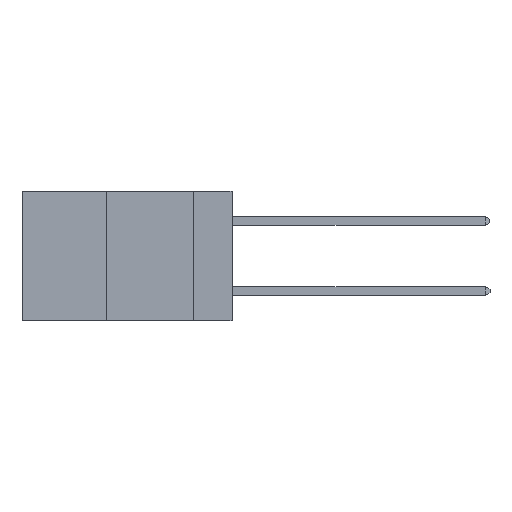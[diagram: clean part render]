
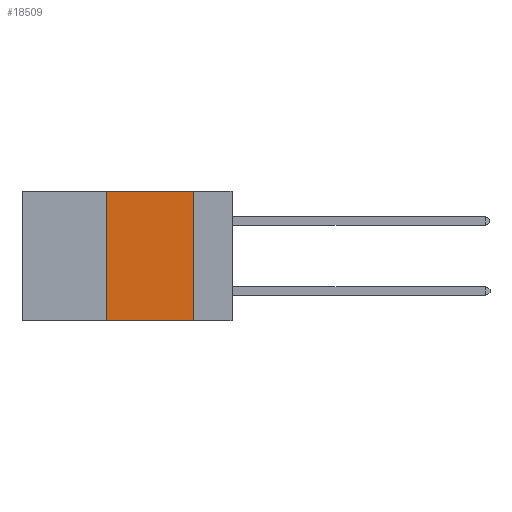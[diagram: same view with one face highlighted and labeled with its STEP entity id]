
A CAD part, left-side view. The second image highlights one B-rep face of the part: STEP entity #18509.
In plain terms, the highlighted planar face has unit normal (-1, 0, 0).
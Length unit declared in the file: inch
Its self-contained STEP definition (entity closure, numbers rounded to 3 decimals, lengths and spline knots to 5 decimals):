
#1529 = EDGE_CURVE ( 'NONE', #11602, #1606, #22416, .T. ) ;
#1606 = VERTEX_POINT ( 'NONE', #14369 ) ;
#1639 = CARTESIAN_POINT ( 'NONE',  ( 0., 0.6, 0. ) ) ;
#1999 = AXIS2_PLACEMENT_3D ( 'NONE', #11808, #15456, #9695 ) ;
#2536 = DIRECTION ( 'NONE',  ( 0., -1., 0. ) ) ;
#2548 = VECTOR ( 'NONE', #16688, 39.37008 ) ;
#2677 = VECTOR ( 'NONE', #16872, 39.37008 ) ;
#2742 = LINE ( 'NONE', #14700, #20110 ) ;
#3551 = ORIENTED_EDGE ( 'NONE', *, *, #13297, .F. ) ;
#3715 = ORIENTED_EDGE ( 'NONE', *, *, #1529, .F. ) ;
#4458 = PLANE ( 'NONE',  #1999 ) ;
#5146 = ORIENTED_EDGE ( 'NONE', *, *, #6043, .T. ) ;
#5927 = CARTESIAN_POINT ( 'NONE',  ( 0., 0.11, 0. ) ) ;
#6043 = EDGE_CURVE ( 'NONE', #11602, #15658, #2742, .T. ) ;
#7690 = VECTOR ( 'NONE', #11779, 39.37008 ) ;
#7703 = FACE_OUTER_BOUND ( 'NONE', #8476, .T. ) ;
#8131 = EDGE_CURVE ( 'NONE', #14094, #15658, #10756, .T. ) ;
#8476 = EDGE_LOOP ( 'NONE', ( #10136, #3551, #3715, #5146 ) ) ;
#9695 = DIRECTION ( 'NONE',  ( 0., 0., -1. ) ) ;
#10136 = ORIENTED_EDGE ( 'NONE', *, *, #8131, .F. ) ;
#10756 = LINE ( 'NONE', #5927, #2677 ) ;
#11602 = VERTEX_POINT ( 'NONE', #12564 ) ;
#11779 = DIRECTION ( 'NONE',  ( 0., 0., 1. ) ) ;
#11801 = LINE ( 'NONE', #1639, #2548 ) ;
#11808 = CARTESIAN_POINT ( 'NONE',  ( 0., 0.6, 0. ) ) ;
#12564 = CARTESIAN_POINT ( 'NONE',  ( 0., 0.36, -0.37 ) ) ;
#13297 = EDGE_CURVE ( 'NONE', #1606, #14094, #11801, .T. ) ;
#14094 = VERTEX_POINT ( 'NONE', #17284 ) ;
#14369 = CARTESIAN_POINT ( 'NONE',  ( 0., 0.36, 0. ) ) ;
#14700 = CARTESIAN_POINT ( 'NONE',  ( 0., 0.6, -0.37 ) ) ;
#15456 = DIRECTION ( 'NONE',  ( 1., 0., 0. ) ) ;
#15658 = VERTEX_POINT ( 'NONE', #23261 ) ;
#16688 = DIRECTION ( 'NONE',  ( 0., -1., 0. ) ) ;
#16872 = DIRECTION ( 'NONE',  ( 0., 0., -1. ) ) ;
#17284 = CARTESIAN_POINT ( 'NONE',  ( 0., 0.11, 0. ) ) ;
#18509 = ADVANCED_FACE ( 'NONE', ( #7703 ), #4458, .F. ) ;
#20110 = VECTOR ( 'NONE', #2536, 39.37008 ) ;
#21089 = CARTESIAN_POINT ( 'NONE',  ( 0., 0.36, 0. ) ) ;
#22416 = LINE ( 'NONE', #21089, #7690 ) ;
#23261 = CARTESIAN_POINT ( 'NONE',  ( 0., 0.11, -0.37 ) ) ;
